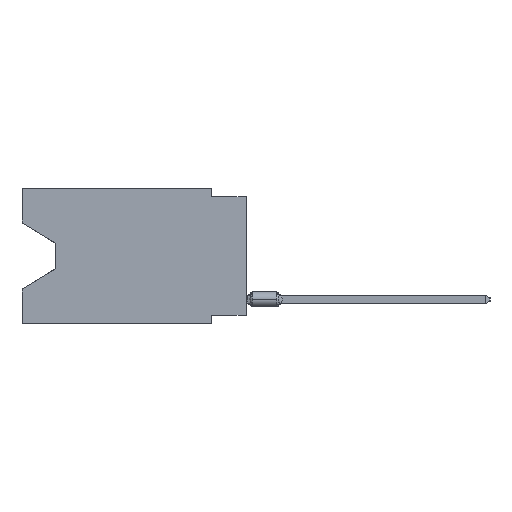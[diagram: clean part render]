
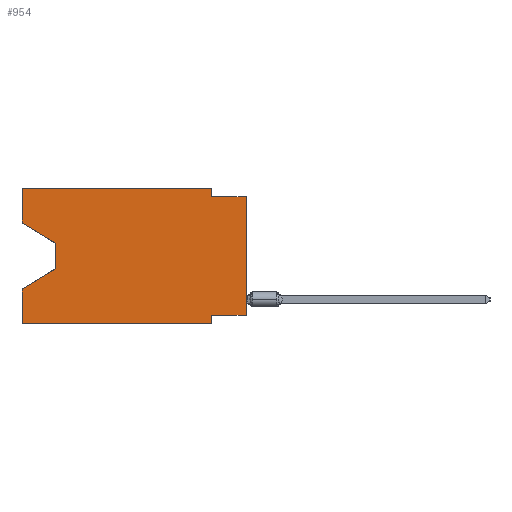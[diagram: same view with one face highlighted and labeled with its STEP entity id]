
A CAD part, left-side view. The second image highlights one B-rep face of the part: STEP entity #954.
In plain terms, the highlighted planar face has unit normal (-1, 0, 0).
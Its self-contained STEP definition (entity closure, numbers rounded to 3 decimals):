
#267 = DIRECTION ( 'NONE',  ( 0., 0., -1. ) ) ;
#290 = AXIS2_PLACEMENT_3D ( 'NONE', #39740, #44242, #267 ) ;
#954 = ADVANCED_FACE ( 'NONE', ( #5086 ), #43928, .F. ) ;
#1501 = DIRECTION ( 'NONE',  ( 0., 0., -1. ) ) ;
#1973 = VECTOR ( 'NONE', #7380, 1000. ) ;
#2554 = ORIENTED_EDGE ( 'NONE', *, *, #6874, .F. ) ;
#3427 = LINE ( 'NONE', #47727, #30890 ) ;
#3584 = LINE ( 'NONE', #23162, #48386 ) ;
#3873 = EDGE_CURVE ( 'NONE', #58670, #14572, #46479, .T. ) ;
#4390 = VERTEX_POINT ( 'NONE', #42978 ) ;
#4890 = ORIENTED_EDGE ( 'NONE', *, *, #42705, .F. ) ;
#5048 = CARTESIAN_POINT ( 'NONE',  ( 0., 16.383, 0. ) ) ;
#5086 = FACE_OUTER_BOUND ( 'NONE', #18617, .T. ) ;
#6408 = VECTOR ( 'NONE', #20135, 1000. ) ;
#6874 = EDGE_CURVE ( 'NONE', #16512, #10815, #60280, .T. ) ;
#6958 = VERTEX_POINT ( 'NONE', #55792 ) ;
#7380 = DIRECTION ( 'NONE',  ( 0., 0., -1. ) ) ;
#7875 = ORIENTED_EDGE ( 'NONE', *, *, #31021, .T. ) ;
#8925 = DIRECTION ( 'NONE',  ( 0., 0., -1. ) ) ;
#10219 = CARTESIAN_POINT ( 'NONE',  ( 0., 16.383, 0. ) ) ;
#10512 = LINE ( 'NONE', #30746, #6408 ) ;
#10815 = VERTEX_POINT ( 'NONE', #22758 ) ;
#10963 = VECTOR ( 'NONE', #37461, 1000. ) ;
#11734 = CARTESIAN_POINT ( 'NONE',  ( 0., 16.383, -7.36 ) ) ;
#12494 = CARTESIAN_POINT ( 'NONE',  ( 0., 13.97, -5.893 ) ) ;
#12938 = ORIENTED_EDGE ( 'NONE', *, *, #22539, .F. ) ;
#13184 = VERTEX_POINT ( 'NONE', #28928 ) ;
#13503 = DIRECTION ( 'NONE',  ( 0., 0., 1. ) ) ;
#13713 = CARTESIAN_POINT ( 'NONE',  ( 0., 0., -9.271 ) ) ;
#14043 = LINE ( 'NONE', #32369, #44914 ) ;
#14207 = VERTEX_POINT ( 'NONE', #12494 ) ;
#14572 = VERTEX_POINT ( 'NONE', #60668 ) ;
#14920 = EDGE_CURVE ( 'NONE', #37140, #13184, #45196, .T. ) ;
#15629 = LINE ( 'NONE', #15940, #17185 ) ;
#15940 = CARTESIAN_POINT ( 'NONE',  ( 0., 2.54, 0. ) ) ;
#16391 = DIRECTION ( 'NONE',  ( 0., -0.855, -0.519 ) ) ;
#16512 = VERTEX_POINT ( 'NONE', #18240 ) ;
#16815 = ORIENTED_EDGE ( 'NONE', *, *, #56428, .T. ) ;
#17146 = VERTEX_POINT ( 'NONE', #11734 ) ;
#17185 = VECTOR ( 'NONE', #1501, 1000. ) ;
#17380 = ORIENTED_EDGE ( 'NONE', *, *, #60679, .T. ) ;
#18240 = CARTESIAN_POINT ( 'NONE',  ( 0., 2.54, -0.635 ) ) ;
#18617 = EDGE_LOOP ( 'NONE', ( #16815, #33296, #17380, #12938, #7875, #47475, #45659, #18957, #2554, #38566, #20642, #4890 ) ) ;
#18957 = ORIENTED_EDGE ( 'NONE', *, *, #46458, .T. ) ;
#20135 = DIRECTION ( 'NONE',  ( 0., 0., 1. ) ) ;
#20642 = ORIENTED_EDGE ( 'NONE', *, *, #14920, .F. ) ;
#22380 = CARTESIAN_POINT ( 'NONE',  ( 0., 0., -9.271 ) ) ;
#22539 = EDGE_CURVE ( 'NONE', #41849, #17146, #10512, .T. ) ;
#22758 = CARTESIAN_POINT ( 'NONE',  ( 0., 0., -0.635 ) ) ;
#23162 = CARTESIAN_POINT ( 'NONE',  ( 0., 0., 0. ) ) ;
#24979 = CARTESIAN_POINT ( 'NONE',  ( 0., 0., -0.635 ) ) ;
#26521 = VECTOR ( 'NONE', #55463, 1000. ) ;
#27475 = DIRECTION ( 'NONE',  ( 0., -1., 0. ) ) ;
#27875 = CARTESIAN_POINT ( 'NONE',  ( 0., 16.383, -9.906 ) ) ;
#28928 = CARTESIAN_POINT ( 'NONE',  ( 0., 2.54, 0. ) ) ;
#30746 = CARTESIAN_POINT ( 'NONE',  ( 0., 16.383, 0. ) ) ;
#30890 = VECTOR ( 'NONE', #16391, 1000. ) ;
#31021 = EDGE_CURVE ( 'NONE', #41849, #37260, #37408, .T. ) ;
#31783 = LINE ( 'NONE', #51366, #1973 ) ;
#32369 = CARTESIAN_POINT ( 'NONE',  ( 0., 2.54, -9.906 ) ) ;
#33149 = LINE ( 'NONE', #52746, #60956 ) ;
#33296 = ORIENTED_EDGE ( 'NONE', *, *, #54897, .T. ) ;
#35018 = DIRECTION ( 'NONE',  ( 0., 0., 1. ) ) ;
#37140 = VERTEX_POINT ( 'NONE', #5048 ) ;
#37260 = VERTEX_POINT ( 'NONE', #61194 ) ;
#37408 = LINE ( 'NONE', #61805, #55020 ) ;
#37461 = DIRECTION ( 'NONE',  ( 0., 1., 0. ) ) ;
#37963 = DIRECTION ( 'NONE',  ( 0., 0.855, -0.519 ) ) ;
#38566 = ORIENTED_EDGE ( 'NONE', *, *, #41534, .F. ) ;
#39740 = CARTESIAN_POINT ( 'NONE',  ( 0., 16.383, 0. ) ) ;
#41534 = EDGE_CURVE ( 'NONE', #13184, #16512, #15629, .T. ) ;
#41849 = VERTEX_POINT ( 'NONE', #27875 ) ;
#41904 = EDGE_CURVE ( 'NONE', #14572, #37260, #14043, .T. ) ;
#42398 = CARTESIAN_POINT ( 'NONE',  ( 0., 16.383, 0. ) ) ;
#42634 = VECTOR ( 'NONE', #63497, 1000. ) ;
#42705 = EDGE_CURVE ( 'NONE', #4390, #37140, #47540, .T. ) ;
#42978 = CARTESIAN_POINT ( 'NONE',  ( 0., 16.383, -2.546 ) ) ;
#43928 = PLANE ( 'NONE',  #290 ) ;
#44242 = DIRECTION ( 'NONE',  ( 1., 0., 0. ) ) ;
#44914 = VECTOR ( 'NONE', #8925, 1000. ) ;
#45196 = LINE ( 'NONE', #10219, #42634 ) ;
#45659 = ORIENTED_EDGE ( 'NONE', *, *, #3873, .F. ) ;
#46458 = EDGE_CURVE ( 'NONE', #58670, #10815, #3584, .T. ) ;
#46479 = LINE ( 'NONE', #22380, #10963 ) ;
#47475 = ORIENTED_EDGE ( 'NONE', *, *, #41904, .F. ) ;
#47540 = LINE ( 'NONE', #42398, #49083 ) ;
#47727 = CARTESIAN_POINT ( 'NONE',  ( 0., 16.383, -2.546 ) ) ;
#48386 = VECTOR ( 'NONE', #35018, 1000. ) ;
#49083 = VECTOR ( 'NONE', #13503, 1000. ) ;
#51366 = CARTESIAN_POINT ( 'NONE',  ( 0., 13.97, -4.013 ) ) ;
#52746 = CARTESIAN_POINT ( 'NONE',  ( 0., 13.97, -5.893 ) ) ;
#54897 = EDGE_CURVE ( 'NONE', #6958, #14207, #31783, .T. ) ;
#55020 = VECTOR ( 'NONE', #27475, 1000. ) ;
#55463 = DIRECTION ( 'NONE',  ( 0., -1., 0. ) ) ;
#55792 = CARTESIAN_POINT ( 'NONE',  ( 0., 13.97, -4.013 ) ) ;
#56428 = EDGE_CURVE ( 'NONE', #4390, #6958, #3427, .T. ) ;
#58670 = VERTEX_POINT ( 'NONE', #13713 ) ;
#60280 = LINE ( 'NONE', #24979, #26521 ) ;
#60668 = CARTESIAN_POINT ( 'NONE',  ( 0., 2.54, -9.271 ) ) ;
#60679 = EDGE_CURVE ( 'NONE', #14207, #17146, #33149, .T. ) ;
#60956 = VECTOR ( 'NONE', #37963, 1000. ) ;
#61194 = CARTESIAN_POINT ( 'NONE',  ( 0., 2.54, -9.906 ) ) ;
#61805 = CARTESIAN_POINT ( 'NONE',  ( 0., 16.383, -9.906 ) ) ;
#63497 = DIRECTION ( 'NONE',  ( 0., -1., 0. ) ) ;
